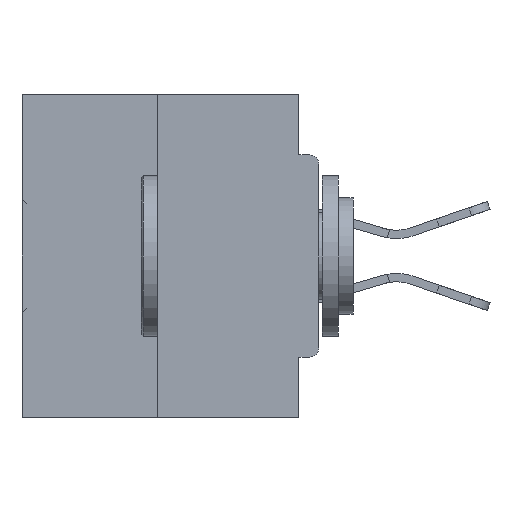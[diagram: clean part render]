
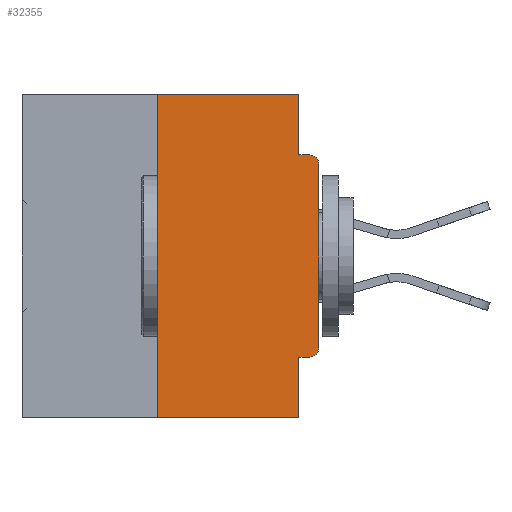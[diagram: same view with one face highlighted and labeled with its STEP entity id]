
A CAD part, left-side view. The second image highlights one B-rep face of the part: STEP entity #32355.
In plain terms, the highlighted planar face has unit normal (-1, 0, 0).
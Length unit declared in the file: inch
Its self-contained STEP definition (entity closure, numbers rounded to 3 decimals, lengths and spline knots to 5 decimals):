
#207 = CARTESIAN_POINT ( 'NONE',  ( 0., 0.031, -0.5 ) ) ;
#232 = DIRECTION ( 'NONE',  ( 0., -1., 0. ) ) ;
#2847 = DIRECTION ( 'NONE',  ( 0., 0., 1. ) ) ;
#2974 = VERTEX_POINT ( 'NONE', #207 ) ;
#3117 = DIRECTION ( 'NONE',  ( 0., 1., 0. ) ) ;
#3700 = CARTESIAN_POINT ( 'NONE',  ( 0., 0.015, -0.0935 ) ) ;
#3953 = VERTEX_POINT ( 'NONE', #3700 ) ;
#5204 = ORIENTED_EDGE ( 'NONE', *, *, #42388, .T. ) ;
#5699 = CARTESIAN_POINT ( 'NONE',  ( 0., 0.031, 0. ) ) ;
#6027 = CARTESIAN_POINT ( 'NONE',  ( 0., 0.031, -0.0935 ) ) ;
#6082 = ORIENTED_EDGE ( 'NONE', *, *, #27883, .F. ) ;
#6105 = DIRECTION ( 'NONE',  ( 0., 0., -1. ) ) ;
#6386 = VERTEX_POINT ( 'NONE', #46535 ) ;
#6427 = CARTESIAN_POINT ( 'NONE',  ( 0., 0.015, -0.1085 ) ) ;
#6905 = LINE ( 'NONE', #23510, #16925 ) ;
#7218 = ORIENTED_EDGE ( 'NONE', *, *, #8863, .F. ) ;
#7509 = ORIENTED_EDGE ( 'NONE', *, *, #41095, .T. ) ;
#7531 = EDGE_LOOP ( 'NONE', ( #7218, #27325, #18527, #6082, #31555, #34481, #5204, #7509, #36938, #29395 ) ) ;
#8863 = EDGE_CURVE ( 'NONE', #16919, #20930, #46393, .T. ) ;
#9586 = CARTESIAN_POINT ( 'NONE',  ( 0., 0.015, -0.3915 ) ) ;
#9752 = CARTESIAN_POINT ( 'NONE',  ( 0., 0.25, 0. ) ) ;
#10347 = CARTESIAN_POINT ( 'NONE',  ( 0., 0.015, -0.4065 ) ) ;
#10371 = VECTOR ( 'NONE', #40111, 39.37008 ) ;
#11239 = CARTESIAN_POINT ( 'NONE',  ( 0., 0.031, 0. ) ) ;
#11789 = CARTESIAN_POINT ( 'NONE',  ( 0., 0.25, 0. ) ) ;
#13040 = CIRCLE ( 'NONE', #36348, 0.015 ) ;
#13163 = DIRECTION ( 'NONE',  ( -1., 0., 0. ) ) ;
#13793 = DIRECTION ( 'NONE',  ( 0., 0., -1. ) ) ;
#14298 = LINE ( 'NONE', #44707, #26146 ) ;
#14470 = CARTESIAN_POINT ( 'NONE',  ( 0., 0.46, 0. ) ) ;
#14938 = VERTEX_POINT ( 'NONE', #6027 ) ;
#15440 = VECTOR ( 'NONE', #28420, 39.37008 ) ;
#15604 = LINE ( 'NONE', #21584, #26666 ) ;
#15735 = LINE ( 'NONE', #29127, #40205 ) ;
#16573 = EDGE_CURVE ( 'NONE', #6386, #16919, #25345, .T. ) ;
#16919 = VERTEX_POINT ( 'NONE', #11789 ) ;
#16925 = VECTOR ( 'NONE', #37956, 39.37008 ) ;
#17757 = CARTESIAN_POINT ( 'NONE',  ( 0., 0., -0.1085 ) ) ;
#17913 = CARTESIAN_POINT ( 'NONE',  ( 0., 0., -0.0935 ) ) ;
#18498 = DIRECTION ( 'NONE',  ( 0., 0., -1. ) ) ;
#18527 = ORIENTED_EDGE ( 'NONE', *, *, #33300, .T. ) ;
#18572 = VERTEX_POINT ( 'NONE', #10347 ) ;
#20392 = VERTEX_POINT ( 'NONE', #17757 ) ;
#20445 = DIRECTION ( 'NONE',  ( 0., 0., -1. ) ) ;
#20930 = VERTEX_POINT ( 'NONE', #11239 ) ;
#21584 = CARTESIAN_POINT ( 'NONE',  ( 0., 0., -0.4065 ) ) ;
#23445 = VECTOR ( 'NONE', #25878, 39.37008 ) ;
#23510 = CARTESIAN_POINT ( 'NONE',  ( 0., 0.031, -0.5 ) ) ;
#24818 = CARTESIAN_POINT ( 'NONE',  ( 0., 0.46, 0. ) ) ;
#25345 = LINE ( 'NONE', #9752, #15440 ) ;
#25878 = DIRECTION ( 'NONE',  ( 0., -1., 0. ) ) ;
#26146 = VECTOR ( 'NONE', #232, 39.37008 ) ;
#26666 = VECTOR ( 'NONE', #3117, 39.37008 ) ;
#27325 = ORIENTED_EDGE ( 'NONE', *, *, #16573, .F. ) ;
#27883 = EDGE_CURVE ( 'NONE', #42860, #2974, #6905, .T. ) ;
#28420 = DIRECTION ( 'NONE',  ( 0., 0., 1. ) ) ;
#29104 = PLANE ( 'NONE',  #34285 ) ;
#29127 = CARTESIAN_POINT ( 'NONE',  ( 0., 0., 0. ) ) ;
#29190 = FACE_OUTER_BOUND ( 'NONE', #7531, .T. ) ;
#29395 = ORIENTED_EDGE ( 'NONE', *, *, #45287, .F. ) ;
#30901 = AXIS2_PLACEMENT_3D ( 'NONE', #9586, #13163, #20445 ) ;
#31555 = ORIENTED_EDGE ( 'NONE', *, *, #47870, .F. ) ;
#31587 = LINE ( 'NONE', #5699, #39680 ) ;
#31740 = EDGE_CURVE ( 'NONE', #14938, #3953, #33348, .T. ) ;
#32355 = ADVANCED_FACE ( 'NONE', ( #29190 ), #29104, .F. ) ;
#32419 = DIRECTION ( 'NONE',  ( -1., 0., 0. ) ) ;
#33300 = EDGE_CURVE ( 'NONE', #6386, #2974, #14298, .T. ) ;
#33348 = LINE ( 'NONE', #17913, #23445 ) ;
#34285 = AXIS2_PLACEMENT_3D ( 'NONE', #14470, #40944, #18498 ) ;
#34481 = ORIENTED_EDGE ( 'NONE', *, *, #45217, .T. ) ;
#36348 = AXIS2_PLACEMENT_3D ( 'NONE', #6427, #32419, #6105 ) ;
#36938 = ORIENTED_EDGE ( 'NONE', *, *, #31740, .F. ) ;
#37956 = DIRECTION ( 'NONE',  ( 0., 0., -1. ) ) ;
#39056 = CARTESIAN_POINT ( 'NONE',  ( 0., 0., -0.3915 ) ) ;
#39680 = VECTOR ( 'NONE', #13793, 39.37008 ) ;
#40111 = DIRECTION ( 'NONE',  ( 0., -1., 0. ) ) ;
#40205 = VECTOR ( 'NONE', #2847, 39.37008 ) ;
#40944 = DIRECTION ( 'NONE',  ( 1., 0., 0. ) ) ;
#41095 = EDGE_CURVE ( 'NONE', #20392, #3953, #13040, .T. ) ;
#42151 = CIRCLE ( 'NONE', #30901, 0.015 ) ;
#42300 = VERTEX_POINT ( 'NONE', #39056 ) ;
#42388 = EDGE_CURVE ( 'NONE', #42300, #20392, #15735, .T. ) ;
#42731 = CARTESIAN_POINT ( 'NONE',  ( 0., 0.031, -0.4065 ) ) ;
#42860 = VERTEX_POINT ( 'NONE', #42731 ) ;
#44707 = CARTESIAN_POINT ( 'NONE',  ( 0., 0.46, -0.5 ) ) ;
#45217 = EDGE_CURVE ( 'NONE', #18572, #42300, #42151, .T. ) ;
#45287 = EDGE_CURVE ( 'NONE', #20930, #14938, #31587, .T. ) ;
#46393 = LINE ( 'NONE', #24818, #10371 ) ;
#46535 = CARTESIAN_POINT ( 'NONE',  ( 0., 0.25, -0.5 ) ) ;
#47870 = EDGE_CURVE ( 'NONE', #18572, #42860, #15604, .T. ) ;
